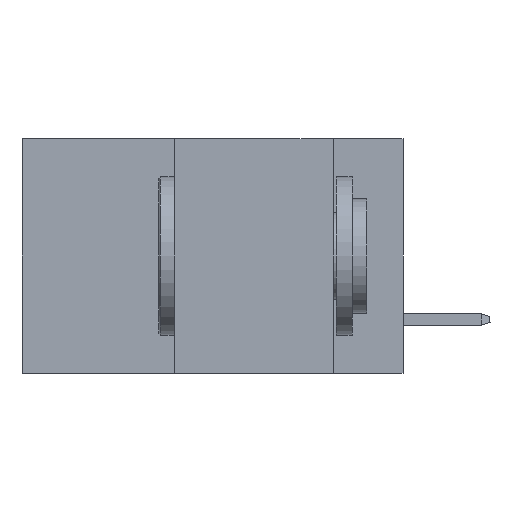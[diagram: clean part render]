
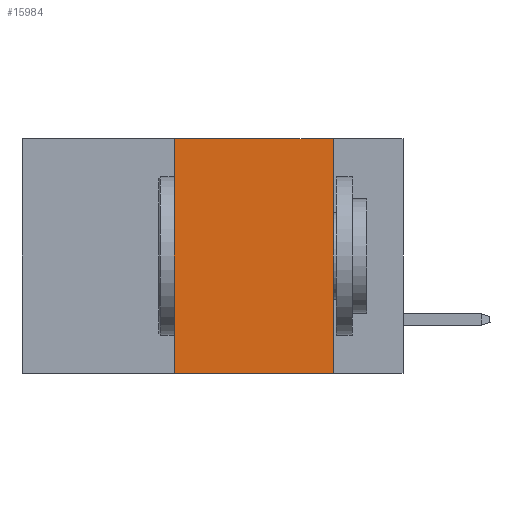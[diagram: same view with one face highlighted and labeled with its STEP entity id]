
A CAD part, left-side view. The second image highlights one B-rep face of the part: STEP entity #15984.
In plain terms, the highlighted planar face has unit normal (-1, 0, 0).
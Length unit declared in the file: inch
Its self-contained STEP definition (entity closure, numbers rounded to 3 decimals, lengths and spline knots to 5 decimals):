
#131 = EDGE_CURVE ( 'NONE', #16682, #29393, #12986, .T. ) ;
#2416 = CARTESIAN_POINT ( 'NONE',  ( 0., 0.11, 0. ) ) ;
#3387 = CARTESIAN_POINT ( 'NONE',  ( 0., 0.36, -0.37 ) ) ;
#4449 = CARTESIAN_POINT ( 'NONE',  ( 0., 0.36, 0. ) ) ;
#5370 = CARTESIAN_POINT ( 'NONE',  ( 0., 0.11, -0.37 ) ) ;
#6331 = DIRECTION ( 'NONE',  ( 0., -1., 0. ) ) ;
#6551 = CARTESIAN_POINT ( 'NONE',  ( 0., 0.6, -0.37 ) ) ;
#6732 = EDGE_LOOP ( 'NONE', ( #13477, #28476, #36901, #14984 ) ) ;
#6762 = PLANE ( 'NONE',  #12615 ) ;
#10079 = EDGE_CURVE ( 'NONE', #18743, #29393, #45421, .T. ) ;
#11306 = LINE ( 'NONE', #18639, #18405 ) ;
#12615 = AXIS2_PLACEMENT_3D ( 'NONE', #20765, #34819, #17324 ) ;
#12986 = LINE ( 'NONE', #2416, #38416 ) ;
#13477 = ORIENTED_EDGE ( 'NONE', *, *, #131, .F. ) ;
#14984 = ORIENTED_EDGE ( 'NONE', *, *, #10079, .T. ) ;
#15984 = ADVANCED_FACE ( 'NONE', ( #38279 ), #6762, .F. ) ;
#16682 = VERTEX_POINT ( 'NONE', #43948 ) ;
#17324 = DIRECTION ( 'NONE',  ( 0., 0., -1. ) ) ;
#18405 = VECTOR ( 'NONE', #32704, 39.37008 ) ;
#18639 = CARTESIAN_POINT ( 'NONE',  ( 0., 0.6, 0. ) ) ;
#18743 = VERTEX_POINT ( 'NONE', #3387 ) ;
#20765 = CARTESIAN_POINT ( 'NONE',  ( 0., 0.6, 0. ) ) ;
#22991 = EDGE_CURVE ( 'NONE', #18743, #30552, #33495, .T. ) ;
#25014 = EDGE_CURVE ( 'NONE', #30552, #16682, #11306, .T. ) ;
#27035 = DIRECTION ( 'NONE',  ( 0., 0., 1. ) ) ;
#28476 = ORIENTED_EDGE ( 'NONE', *, *, #25014, .F. ) ;
#29393 = VERTEX_POINT ( 'NONE', #5370 ) ;
#29803 = CARTESIAN_POINT ( 'NONE',  ( 0., 0.36, 0. ) ) ;
#30552 = VERTEX_POINT ( 'NONE', #4449 ) ;
#32244 = VECTOR ( 'NONE', #27035, 39.37008 ) ;
#32704 = DIRECTION ( 'NONE',  ( 0., -1., 0. ) ) ;
#32708 = VECTOR ( 'NONE', #6331, 39.37008 ) ;
#33495 = LINE ( 'NONE', #29803, #32244 ) ;
#34365 = DIRECTION ( 'NONE',  ( 0., 0., -1. ) ) ;
#34819 = DIRECTION ( 'NONE',  ( 1., 0., 0. ) ) ;
#36901 = ORIENTED_EDGE ( 'NONE', *, *, #22991, .F. ) ;
#38279 = FACE_OUTER_BOUND ( 'NONE', #6732, .T. ) ;
#38416 = VECTOR ( 'NONE', #34365, 39.37008 ) ;
#43948 = CARTESIAN_POINT ( 'NONE',  ( 0., 0.11, 0. ) ) ;
#45421 = LINE ( 'NONE', #6551, #32708 ) ;
